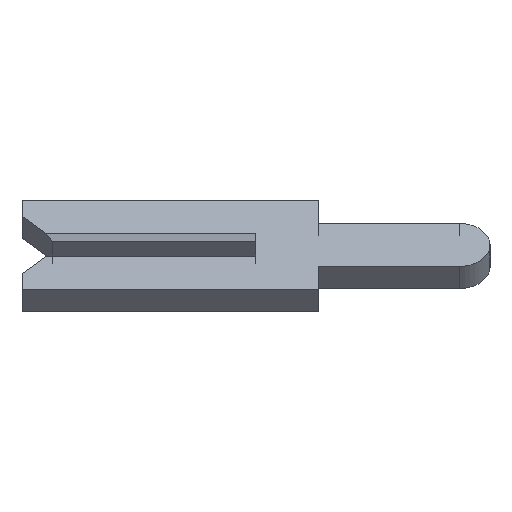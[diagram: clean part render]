
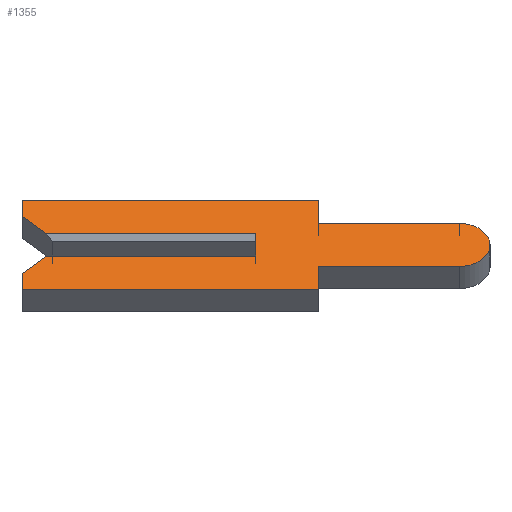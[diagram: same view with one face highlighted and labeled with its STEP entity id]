
A CAD part, left-side view. The second image highlights one B-rep face of the part: STEP entity #1355.
In plain terms, the highlighted face is planar.
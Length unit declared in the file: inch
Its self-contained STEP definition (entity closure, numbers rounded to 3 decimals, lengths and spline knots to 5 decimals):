
#15 = LINE ( 'NONE', #62, #1038 ) ;
#17 = DIRECTION ( 'NONE',  ( 1., 0., 0. ) ) ;
#39 = CARTESIAN_POINT ( 'NONE',  ( -0.01, 0., -0.01 ) ) ;
#50 = ORIENTED_EDGE ( 'NONE', *, *, #466, .F. ) ;
#57 = EDGE_CURVE ( 'NONE', #1163, #619, #1391, .T. ) ;
#62 = CARTESIAN_POINT ( 'NONE',  ( -0.01, -0.04, 0.0195 ) ) ;
#67 = EDGE_LOOP ( 'NONE', ( #553, #442, #1264, #475, #189, #254, #874, #1262, #208, #853, #50, #223, #811, #147 ) ) ;
#88 = EDGE_CURVE ( 'NONE', #976, #887, #832, .T. ) ;
#95 = FACE_OUTER_BOUND ( 'NONE', #67, .T. ) ;
#98 = VERTEX_POINT ( 'NONE', #1135 ) ;
#103 = CARTESIAN_POINT ( 'NONE',  ( -0.01, 0., 0.0065 ) ) ;
#114 = EDGE_CURVE ( 'NONE', #547, #241, #834, .T. ) ;
#145 = CARTESIAN_POINT ( 'NONE',  ( -0.01, -0.04, -0.04 ) ) ;
#147 = ORIENTED_EDGE ( 'NONE', *, *, #1003, .F. ) ;
#151 = LINE ( 'NONE', #991, #1336 ) ;
#154 = CIRCLE ( 'NONE', #281, 0.0195 ) ;
#158 = DIRECTION ( 'NONE',  ( 0., 0., -1. ) ) ;
#189 = ORIENTED_EDGE ( 'NONE', *, *, #1269, .F. ) ;
#208 = ORIENTED_EDGE ( 'NONE', *, *, #211, .F. ) ;
#211 = EDGE_CURVE ( 'NONE', #98, #855, #154, .T. ) ;
#212 = DIRECTION ( 'NONE',  ( 0., -1., 0. ) ) ;
#223 = ORIENTED_EDGE ( 'NONE', *, *, #333, .F. ) ;
#241 = VERTEX_POINT ( 'NONE', #250 ) ;
#250 = CARTESIAN_POINT ( 'NONE',  ( -0.01, 0.15, -0.04 ) ) ;
#254 = ORIENTED_EDGE ( 'NONE', *, *, #114, .F. ) ;
#270 = DIRECTION ( 'NONE',  ( 0., 0., -1. ) ) ;
#281 = AXIS2_PLACEMENT_3D ( 'NONE', #451, #17, #928 ) ;
#301 = CARTESIAN_POINT ( 'NONE',  ( -0.01, 0., 0.01 ) ) ;
#333 = EDGE_CURVE ( 'NONE', #1249, #1146, #1017, .T. ) ;
#340 = CARTESIAN_POINT ( 'NONE',  ( -0.01, 0.15, -0.026 ) ) ;
#358 = LINE ( 'NONE', #422, #495 ) ;
#362 = VECTOR ( 'NONE', #673, 39.37008 ) ;
#371 = CARTESIAN_POINT ( 'NONE',  ( -0.01, -0.04, 0.04 ) ) ;
#388 = CARTESIAN_POINT ( 'NONE',  ( -0.01, -0.04, -0.04 ) ) ;
#399 = VECTOR ( 'NONE', #1401, 39.37008 ) ;
#401 = CARTESIAN_POINT ( 'NONE',  ( -0.01, -0.04, 0.0195 ) ) ;
#420 = PLANE ( 'NONE',  #542 ) ;
#422 = CARTESIAN_POINT ( 'NONE',  ( -0.01, 0.1305, -0.0065 ) ) ;
#430 = LINE ( 'NONE', #837, #399 ) ;
#431 = CARTESIAN_POINT ( 'NONE',  ( -0.01, 0.15, 0.026 ) ) ;
#442 = ORIENTED_EDGE ( 'NONE', *, *, #1318, .F. ) ;
#451 = CARTESIAN_POINT ( 'NONE',  ( -0.01, -0.1305, 0. ) ) ;
#452 = EDGE_CURVE ( 'NONE', #583, #547, #598, .T. ) ;
#455 = LINE ( 'NONE', #371, #867 ) ;
#466 = EDGE_CURVE ( 'NONE', #1146, #1104, #455, .T. ) ;
#475 = ORIENTED_EDGE ( 'NONE', *, *, #1275, .F. ) ;
#492 = CARTESIAN_POINT ( 'NONE',  ( -0.01, -0.04, -0.0195 ) ) ;
#495 = VECTOR ( 'NONE', #1216, 39.37008 ) ;
#503 = DIRECTION ( 'NONE',  ( 0., 0.707, 0.707 ) ) ;
#529 = VECTOR ( 'NONE', #212, 39.37008 ) ;
#531 = VECTOR ( 'NONE', #791, 39.37008 ) ;
#542 = AXIS2_PLACEMENT_3D ( 'NONE', #1338, #1352, #789 ) ;
#543 = DIRECTION ( 'NONE',  ( 0., -1., 0. ) ) ;
#547 = VERTEX_POINT ( 'NONE', #388 ) ;
#553 = ORIENTED_EDGE ( 'NONE', *, *, #88, .T. ) ;
#583 = VERTEX_POINT ( 'NONE', #492 ) ;
#598 = LINE ( 'NONE', #145, #1064 ) ;
#615 = LINE ( 'NONE', #103, #1032 ) ;
#619 = VERTEX_POINT ( 'NONE', #39 ) ;
#624 = EDGE_CURVE ( 'NONE', #855, #583, #430, .T. ) ;
#627 = CARTESIAN_POINT ( 'NONE',  ( -0.01, 0.134, 0.01 ) ) ;
#645 = CARTESIAN_POINT ( 'NONE',  ( -0.01, -0.04, 0.04 ) ) ;
#647 = CARTESIAN_POINT ( 'NONE',  ( -0.01, 0.15, -0.04 ) ) ;
#673 = DIRECTION ( 'NONE',  ( 0., -1., 0. ) ) ;
#746 = CARTESIAN_POINT ( 'NONE',  ( -0.01, 0.1305, 0.0065 ) ) ;
#789 = DIRECTION ( 'NONE',  ( 0., 0., -1. ) ) ;
#791 = DIRECTION ( 'NONE',  ( 0., 1., 0. ) ) ;
#811 = ORIENTED_EDGE ( 'NONE', *, *, #1113, .F. ) ;
#832 = LINE ( 'NONE', #898, #995 ) ;
#834 = LINE ( 'NONE', #647, #531 ) ;
#837 = CARTESIAN_POINT ( 'NONE',  ( -0.01, -0.04, -0.0195 ) ) ;
#838 = LINE ( 'NONE', #746, #1375 ) ;
#843 = DIRECTION ( 'NONE',  ( 0., 0., 1. ) ) ;
#851 = DIRECTION ( 'NONE',  ( 0., -1., 0. ) ) ;
#853 = ORIENTED_EDGE ( 'NONE', *, *, #894, .F. ) ;
#855 = VERTEX_POINT ( 'NONE', #1197 ) ;
#867 = VECTOR ( 'NONE', #158, 39.37008 ) ;
#873 = CARTESIAN_POINT ( 'NONE',  ( -0.01, 0.134, -0.01 ) ) ;
#874 = ORIENTED_EDGE ( 'NONE', *, *, #452, .F. ) ;
#879 = DIRECTION ( 'NONE',  ( 0., 0., 1. ) ) ;
#887 = VERTEX_POINT ( 'NONE', #301 ) ;
#894 = EDGE_CURVE ( 'NONE', #1104, #98, #15, .T. ) ;
#898 = CARTESIAN_POINT ( 'NONE',  ( -0.01, 0.15, 0.01 ) ) ;
#928 = DIRECTION ( 'NONE',  ( 0., 0., -1. ) ) ;
#976 = VERTEX_POINT ( 'NONE', #627 ) ;
#991 = CARTESIAN_POINT ( 'NONE',  ( -0.01, 0.15, -0.026 ) ) ;
#995 = VECTOR ( 'NONE', #543, 39.37008 ) ;
#998 = CARTESIAN_POINT ( 'NONE',  ( -0.01, 0.15, 0.04 ) ) ;
#1003 = EDGE_CURVE ( 'NONE', #976, #1226, #838, .T. ) ;
#1017 = LINE ( 'NONE', #1026, #362 ) ;
#1026 = CARTESIAN_POINT ( 'NONE',  ( -0.01, 0.15, 0.04 ) ) ;
#1032 = VECTOR ( 'NONE', #1217, 39.37008 ) ;
#1038 = VECTOR ( 'NONE', #851, 39.37008 ) ;
#1064 = VECTOR ( 'NONE', #270, 39.37008 ) ;
#1104 = VERTEX_POINT ( 'NONE', #401 ) ;
#1113 = EDGE_CURVE ( 'NONE', #1226, #1249, #1281, .T. ) ;
#1126 = CARTESIAN_POINT ( 'NONE',  ( -0.01, -0.1305, -0.01 ) ) ;
#1135 = CARTESIAN_POINT ( 'NONE',  ( -0.01, -0.1305, 0.0195 ) ) ;
#1146 = VERTEX_POINT ( 'NONE', #645 ) ;
#1163 = VERTEX_POINT ( 'NONE', #873 ) ;
#1197 = CARTESIAN_POINT ( 'NONE',  ( -0.01, -0.1305, -0.0195 ) ) ;
#1216 = DIRECTION ( 'NONE',  ( 0., -0.707, 0.707 ) ) ;
#1217 = DIRECTION ( 'NONE',  ( 0., 0., 1. ) ) ;
#1226 = VERTEX_POINT ( 'NONE', #431 ) ;
#1249 = VERTEX_POINT ( 'NONE', #998 ) ;
#1262 = ORIENTED_EDGE ( 'NONE', *, *, #624, .F. ) ;
#1264 = ORIENTED_EDGE ( 'NONE', *, *, #57, .F. ) ;
#1269 = EDGE_CURVE ( 'NONE', #241, #1374, #151, .T. ) ;
#1275 = EDGE_CURVE ( 'NONE', #1374, #1163, #358, .T. ) ;
#1281 = LINE ( 'NONE', #1310, #1299 ) ;
#1299 = VECTOR ( 'NONE', #843, 39.37008 ) ;
#1310 = CARTESIAN_POINT ( 'NONE',  ( -0.01, 0.15, 0.026 ) ) ;
#1318 = EDGE_CURVE ( 'NONE', #619, #887, #615, .T. ) ;
#1336 = VECTOR ( 'NONE', #879, 39.37008 ) ;
#1338 = CARTESIAN_POINT ( 'NONE',  ( -0.01, -0.1305, 0. ) ) ;
#1352 = DIRECTION ( 'NONE',  ( 1., 0., 0. ) ) ;
#1355 = ADVANCED_FACE ( 'NONE', ( #95 ), #420, .F. ) ;
#1374 = VERTEX_POINT ( 'NONE', #340 ) ;
#1375 = VECTOR ( 'NONE', #503, 39.37008 ) ;
#1391 = LINE ( 'NONE', #1126, #529 ) ;
#1401 = DIRECTION ( 'NONE',  ( 0., 1., 0. ) ) ;
